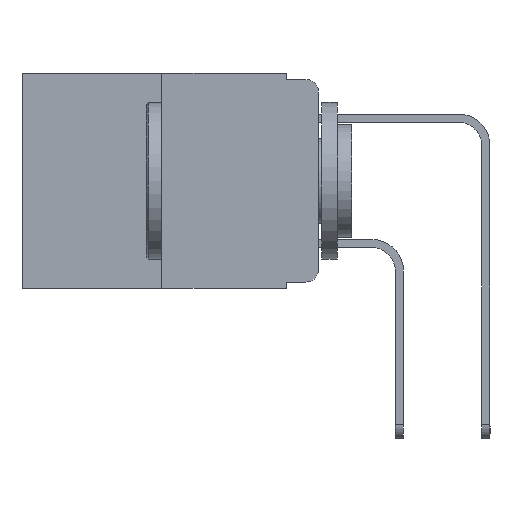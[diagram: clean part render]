
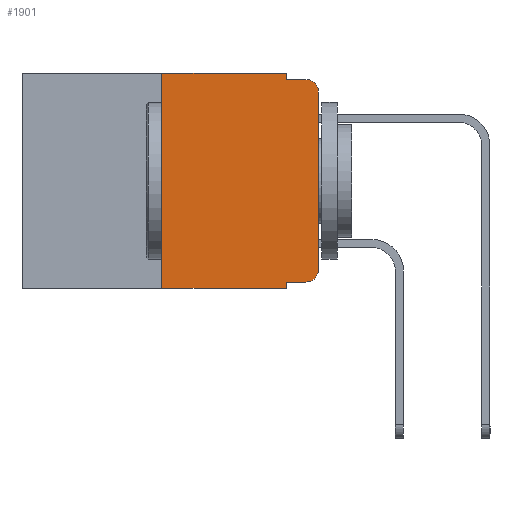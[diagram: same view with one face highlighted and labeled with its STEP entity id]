
A CAD part, left-side view. The second image highlights one B-rep face of the part: STEP entity #1901.
In plain terms, the highlighted planar face has unit normal (-1, 0, 0).
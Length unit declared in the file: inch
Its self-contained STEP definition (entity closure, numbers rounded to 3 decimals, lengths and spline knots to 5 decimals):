
#135 = CARTESIAN_POINT ( 'NONE',  ( 0., 0., 0. ) ) ;
#168 = EDGE_CURVE ( 'NONE', #11497, #6330, #4824, .T. ) ;
#440 = CARTESIAN_POINT ( 'NONE',  ( 0., 0.051, -0.333 ) ) ;
#519 = ORIENTED_EDGE ( 'NONE', *, *, #5920, .T. ) ;
#558 = DIRECTION ( 'NONE',  ( 0., -1., 0. ) ) ;
#835 = CARTESIAN_POINT ( 'NONE',  ( 0., 0.051, 0. ) ) ;
#896 = VECTOR ( 'NONE', #5828, 39.37008 ) ;
#976 = CARTESIAN_POINT ( 'NONE',  ( 0., 0.02, -0.333 ) ) ;
#1175 = DIRECTION ( 'NONE',  ( 0., 0., -1. ) ) ;
#1440 = LINE ( 'NONE', #135, #896 ) ;
#1481 = CIRCLE ( 'NONE', #13992, 0.02 ) ;
#1749 = DIRECTION ( 'NONE',  ( 1., 0., 0. ) ) ;
#1901 = ADVANCED_FACE ( 'NONE', ( #3160 ), #8830, .F. ) ;
#1955 = LINE ( 'NONE', #7637, #2695 ) ;
#1957 = LINE ( 'NONE', #7641, #8381 ) ;
#2111 = ORIENTED_EDGE ( 'NONE', *, *, #6392, .F. ) ;
#2624 = VERTEX_POINT ( 'NONE', #14186 ) ;
#2648 = ORIENTED_EDGE ( 'NONE', *, *, #4165, .F. ) ;
#2686 = CARTESIAN_POINT ( 'NONE',  ( 0., 0.051, -0.01 ) ) ;
#2695 = VECTOR ( 'NONE', #558, 39.37008 ) ;
#2930 = VERTEX_POINT ( 'NONE', #2686 ) ;
#3160 = FACE_OUTER_BOUND ( 'NONE', #16353, .T. ) ;
#3276 = DIRECTION ( 'NONE',  ( 0., -1., 0. ) ) ;
#3498 = CARTESIAN_POINT ( 'NONE',  ( 0., 0.25, -0.343 ) ) ;
#4165 = EDGE_CURVE ( 'NONE', #18311, #2624, #6569, .T. ) ;
#4588 = CARTESIAN_POINT ( 'NONE',  ( 0., 0.473, 0. ) ) ;
#4703 = CARTESIAN_POINT ( 'NONE',  ( 0., 0.051, -0.333 ) ) ;
#4824 = LINE ( 'NONE', #10517, #13112 ) ;
#5036 = ORIENTED_EDGE ( 'NONE', *, *, #14029, .T. ) ;
#5129 = LINE ( 'NONE', #835, #12197 ) ;
#5424 = CARTESIAN_POINT ( 'NONE',  ( 0., 0., -0.313 ) ) ;
#5729 = DIRECTION ( 'NONE',  ( 0., 0., -1. ) ) ;
#5828 = DIRECTION ( 'NONE',  ( 0., 0., 1. ) ) ;
#5920 = EDGE_CURVE ( 'NONE', #11497, #8032, #14688, .T. ) ;
#6149 = VERTEX_POINT ( 'NONE', #5424 ) ;
#6318 = CARTESIAN_POINT ( 'NONE',  ( 0., 0.051, 0. ) ) ;
#6330 = VERTEX_POINT ( 'NONE', #11945 ) ;
#6392 = EDGE_CURVE ( 'NONE', #2624, #16096, #13061, .T. ) ;
#6569 = LINE ( 'NONE', #11057, #9833 ) ;
#6580 = CARTESIAN_POINT ( 'NONE',  ( 0., 0.02, -0.03 ) ) ;
#6699 = DIRECTION ( 'NONE',  ( 0., 0., -1. ) ) ;
#6945 = CARTESIAN_POINT ( 'NONE',  ( 0., 0.02, -0.313 ) ) ;
#7130 = AXIS2_PLACEMENT_3D ( 'NONE', #14540, #1749, #7434 ) ;
#7434 = DIRECTION ( 'NONE',  ( 0., 0., -1. ) ) ;
#7513 = EDGE_CURVE ( 'NONE', #10717, #8225, #1481, .T. ) ;
#7637 = CARTESIAN_POINT ( 'NONE',  ( 0., 0.473, -0.343 ) ) ;
#7641 = CARTESIAN_POINT ( 'NONE',  ( 0., 0.051, -0.01 ) ) ;
#7981 = DIRECTION ( 'NONE',  ( -1., 0., 0. ) ) ;
#8032 = VERTEX_POINT ( 'NONE', #976 ) ;
#8225 = VERTEX_POINT ( 'NONE', #8401 ) ;
#8381 = VECTOR ( 'NONE', #3276, 39.37008 ) ;
#8392 = EDGE_CURVE ( 'NONE', #16096, #2930, #5129, .T. ) ;
#8401 = CARTESIAN_POINT ( 'NONE',  ( 0., 0.02, -0.01 ) ) ;
#8586 = CARTESIAN_POINT ( 'NONE',  ( 0., 0., -0.03 ) ) ;
#8830 = PLANE ( 'NONE',  #7130 ) ;
#9073 = EDGE_CURVE ( 'NONE', #6149, #10717, #1440, .T. ) ;
#9780 = ORIENTED_EDGE ( 'NONE', *, *, #9073, .T. ) ;
#9833 = VECTOR ( 'NONE', #12169, 39.37008 ) ;
#10077 = EDGE_CURVE ( 'NONE', #18311, #6330, #1955, .T. ) ;
#10363 = ORIENTED_EDGE ( 'NONE', *, *, #8392, .F. ) ;
#10517 = CARTESIAN_POINT ( 'NONE',  ( 0., 0.051, 0. ) ) ;
#10717 = VERTEX_POINT ( 'NONE', #8586 ) ;
#11057 = CARTESIAN_POINT ( 'NONE',  ( 0., 0.25, 0. ) ) ;
#11269 = EDGE_CURVE ( 'NONE', #2930, #8225, #1957, .T. ) ;
#11497 = VERTEX_POINT ( 'NONE', #440 ) ;
#11945 = CARTESIAN_POINT ( 'NONE',  ( 0., 0.051, -0.343 ) ) ;
#12169 = DIRECTION ( 'NONE',  ( 0., 0., 1. ) ) ;
#12197 = VECTOR ( 'NONE', #6699, 39.37008 ) ;
#12619 = ORIENTED_EDGE ( 'NONE', *, *, #168, .F. ) ;
#12673 = ORIENTED_EDGE ( 'NONE', *, *, #10077, .T. ) ;
#13061 = LINE ( 'NONE', #4588, #14562 ) ;
#13112 = VECTOR ( 'NONE', #1175, 39.37008 ) ;
#13672 = DIRECTION ( 'NONE',  ( 0., 0., -1. ) ) ;
#13992 = AXIS2_PLACEMENT_3D ( 'NONE', #6580, #7981, #13672 ) ;
#14029 = EDGE_CURVE ( 'NONE', #8032, #6149, #14971, .T. ) ;
#14186 = CARTESIAN_POINT ( 'NONE',  ( 0., 0.25, 0. ) ) ;
#14540 = CARTESIAN_POINT ( 'NONE',  ( 0., 0.473, 0. ) ) ;
#14562 = VECTOR ( 'NONE', #15972, 39.37008 ) ;
#14688 = LINE ( 'NONE', #4703, #18135 ) ;
#14779 = DIRECTION ( 'NONE',  ( 0., -1., 0. ) ) ;
#14971 = CIRCLE ( 'NONE', #17960, 0.02 ) ;
#15972 = DIRECTION ( 'NONE',  ( 0., -1., 0. ) ) ;
#16096 = VERTEX_POINT ( 'NONE', #6318 ) ;
#16353 = EDGE_LOOP ( 'NONE', ( #9780, #18271, #17705, #10363, #2111, #2648, #12673, #12619, #519, #5036 ) ) ;
#17705 = ORIENTED_EDGE ( 'NONE', *, *, #11269, .F. ) ;
#17960 = AXIS2_PLACEMENT_3D ( 'NONE', #6945, #18326, #5729 ) ;
#18135 = VECTOR ( 'NONE', #14779, 39.37008 ) ;
#18271 = ORIENTED_EDGE ( 'NONE', *, *, #7513, .T. ) ;
#18311 = VERTEX_POINT ( 'NONE', #3498 ) ;
#18326 = DIRECTION ( 'NONE',  ( -1., 0., 0. ) ) ;
